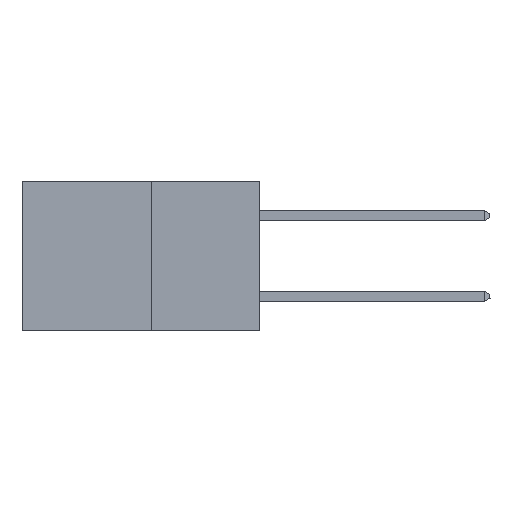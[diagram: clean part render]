
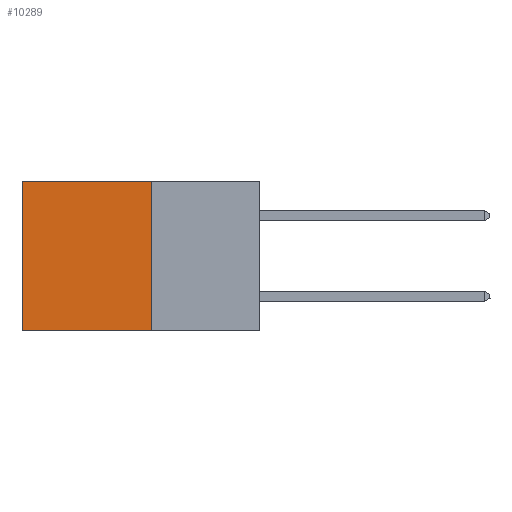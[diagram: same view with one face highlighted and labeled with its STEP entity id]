
A CAD part, left-side view. The second image highlights one B-rep face of the part: STEP entity #10289.
In plain terms, the highlighted planar face has unit normal (-1, 0, 0).
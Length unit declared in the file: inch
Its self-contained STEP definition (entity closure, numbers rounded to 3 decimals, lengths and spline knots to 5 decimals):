
#351 = CARTESIAN_POINT ( 'NONE',  ( 0.277, 0.27, -0.37 ) ) ;
#670 = VECTOR ( 'NONE', #21270, 39.37008 ) ;
#711 = CARTESIAN_POINT ( 'NONE',  ( 0.277, 0.59, -0.37 ) ) ;
#1025 = CARTESIAN_POINT ( 'NONE',  ( 0.277, 0.27, 0. ) ) ;
#1481 = VECTOR ( 'NONE', #21912, 39.37008 ) ;
#3666 = VECTOR ( 'NONE', #20296, 39.37008 ) ;
#4353 = EDGE_LOOP ( 'NONE', ( #28837, #33001, #23766, #24988 ) ) ;
#4927 = FACE_OUTER_BOUND ( 'NONE', #4353, .T. ) ;
#5384 = VECTOR ( 'NONE', #21521, 39.37008 ) ;
#6538 = CARTESIAN_POINT ( 'NONE',  ( 0.277, 0.27, 0. ) ) ;
#7493 = VERTEX_POINT ( 'NONE', #14622 ) ;
#8521 = LINE ( 'NONE', #351, #670 ) ;
#10289 = ADVANCED_FACE ( 'NONE', ( #4927 ), #19162, .F. ) ;
#10576 = EDGE_CURVE ( 'NONE', #7493, #11677, #10650, .T. ) ;
#10650 = LINE ( 'NONE', #25416, #3666 ) ;
#11452 = DIRECTION ( 'NONE',  ( 1., 0., 0. ) ) ;
#11524 = LINE ( 'NONE', #18882, #5384 ) ;
#11677 = VERTEX_POINT ( 'NONE', #711 ) ;
#13417 = CARTESIAN_POINT ( 'NONE',  ( 0.277, 0.27, -0.37 ) ) ;
#14473 = AXIS2_PLACEMENT_3D ( 'NONE', #27044, #11452, #29670 ) ;
#14622 = CARTESIAN_POINT ( 'NONE',  ( 0.277, 0.59, 0. ) ) ;
#16218 = LINE ( 'NONE', #1025, #1481 ) ;
#18882 = CARTESIAN_POINT ( 'NONE',  ( 0.277, 0.27, -0.37 ) ) ;
#18910 = EDGE_CURVE ( 'NONE', #21835, #7493, #16218, .T. ) ;
#19162 = PLANE ( 'NONE',  #14473 ) ;
#19579 = VERTEX_POINT ( 'NONE', #13417 ) ;
#20296 = DIRECTION ( 'NONE',  ( 0., 0., -1. ) ) ;
#21270 = DIRECTION ( 'NONE',  ( 0., 0., -1. ) ) ;
#21521 = DIRECTION ( 'NONE',  ( 0., 1., 0. ) ) ;
#21835 = VERTEX_POINT ( 'NONE', #6538 ) ;
#21912 = DIRECTION ( 'NONE',  ( 0., 1., 0. ) ) ;
#23766 = ORIENTED_EDGE ( 'NONE', *, *, #26642, .F. ) ;
#24988 = ORIENTED_EDGE ( 'NONE', *, *, #18910, .T. ) ;
#25416 = CARTESIAN_POINT ( 'NONE',  ( 0.277, 0.59, -0.37 ) ) ;
#26642 = EDGE_CURVE ( 'NONE', #21835, #19579, #8521, .T. ) ;
#27044 = CARTESIAN_POINT ( 'NONE',  ( 0.277, 0.27, -0.37 ) ) ;
#28155 = EDGE_CURVE ( 'NONE', #19579, #11677, #11524, .T. ) ;
#28837 = ORIENTED_EDGE ( 'NONE', *, *, #10576, .T. ) ;
#29670 = DIRECTION ( 'NONE',  ( 0., 0., -1. ) ) ;
#33001 = ORIENTED_EDGE ( 'NONE', *, *, #28155, .F. ) ;
